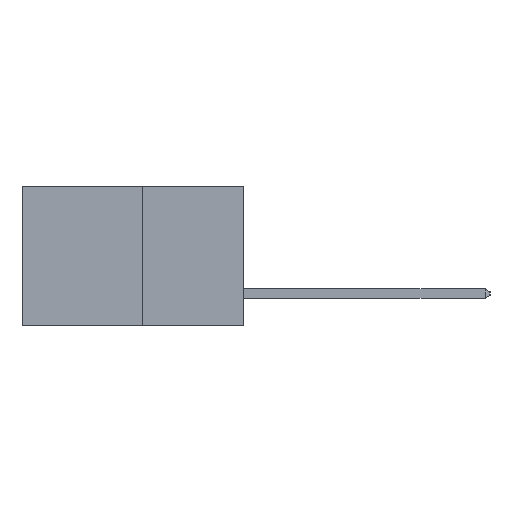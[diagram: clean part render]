
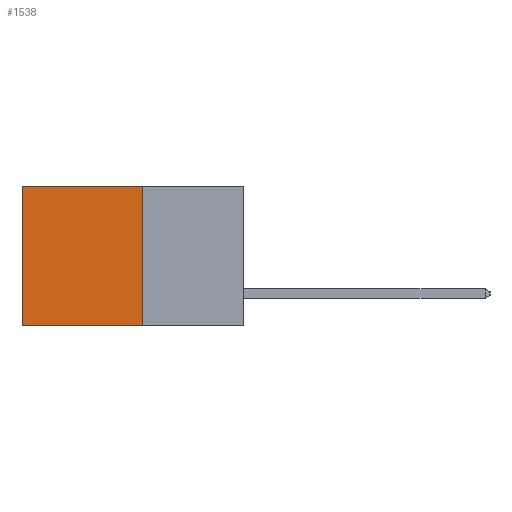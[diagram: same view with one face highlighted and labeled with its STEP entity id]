
A CAD part, left-side view. The second image highlights one B-rep face of the part: STEP entity #1538.
In plain terms, the highlighted planar face has unit normal (-1, 0, 0).
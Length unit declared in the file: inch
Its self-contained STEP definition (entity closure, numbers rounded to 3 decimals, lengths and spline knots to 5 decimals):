
#100 = LINE ( 'NONE', #8875, #11781 ) ;
#270 = CARTESIAN_POINT ( 'NONE',  ( 0.277, 0.27, -0.37 ) ) ;
#289 = CARTESIAN_POINT ( 'NONE',  ( 0.277, 0.59, -0.37 ) ) ;
#321 = DIRECTION ( 'NONE',  ( 0., 1., 0. ) ) ;
#931 = CARTESIAN_POINT ( 'NONE',  ( 0.277, 0.59, 0. ) ) ;
#1231 = CARTESIAN_POINT ( 'NONE',  ( 0.277, 0.27, 0. ) ) ;
#1324 = VERTEX_POINT ( 'NONE', #289 ) ;
#1538 = ADVANCED_FACE ( 'NONE', ( #3487 ), #2249, .F. ) ;
#2160 = CARTESIAN_POINT ( 'NONE',  ( 0.277, 0.27, -0.37 ) ) ;
#2249 = PLANE ( 'NONE',  #11207 ) ;
#3296 = ORIENTED_EDGE ( 'NONE', *, *, #9371, .T. ) ;
#3473 = CARTESIAN_POINT ( 'NONE',  ( 0.277, 0.27, -0.37 ) ) ;
#3487 = FACE_OUTER_BOUND ( 'NONE', #5693, .T. ) ;
#3589 = DIRECTION ( 'NONE',  ( 0., 0., -1. ) ) ;
#3877 = CARTESIAN_POINT ( 'NONE',  ( 0.277, 0.27, 0. ) ) ;
#3900 = DIRECTION ( 'NONE',  ( 0., 0., -1. ) ) ;
#5597 = DIRECTION ( 'NONE',  ( 1., 0., 0. ) ) ;
#5641 = EDGE_CURVE ( 'NONE', #7639, #1324, #5651, .T. ) ;
#5651 = LINE ( 'NONE', #270, #10598 ) ;
#5693 = EDGE_LOOP ( 'NONE', ( #3296, #5935, #12769, #12061 ) ) ;
#5935 = ORIENTED_EDGE ( 'NONE', *, *, #5641, .F. ) ;
#6694 = EDGE_CURVE ( 'NONE', #10848, #10465, #9788, .T. ) ;
#6961 = VECTOR ( 'NONE', #9824, 39.37008 ) ;
#7639 = VERTEX_POINT ( 'NONE', #9329 ) ;
#8875 = CARTESIAN_POINT ( 'NONE',  ( 0.277, 0.59, -0.37 ) ) ;
#9329 = CARTESIAN_POINT ( 'NONE',  ( 0.277, 0.27, -0.37 ) ) ;
#9371 = EDGE_CURVE ( 'NONE', #10465, #1324, #100, .T. ) ;
#9771 = DIRECTION ( 'NONE',  ( 0., 1., 0. ) ) ;
#9788 = LINE ( 'NONE', #1231, #10754 ) ;
#9824 = DIRECTION ( 'NONE',  ( 0., 0., -1. ) ) ;
#10465 = VERTEX_POINT ( 'NONE', #931 ) ;
#10598 = VECTOR ( 'NONE', #321, 39.37008 ) ;
#10754 = VECTOR ( 'NONE', #9771, 39.37008 ) ;
#10848 = VERTEX_POINT ( 'NONE', #3877 ) ;
#11207 = AXIS2_PLACEMENT_3D ( 'NONE', #2160, #5597, #3900 ) ;
#11781 = VECTOR ( 'NONE', #3589, 39.37008 ) ;
#12061 = ORIENTED_EDGE ( 'NONE', *, *, #6694, .T. ) ;
#12494 = LINE ( 'NONE', #3473, #6961 ) ;
#12769 = ORIENTED_EDGE ( 'NONE', *, *, #13177, .F. ) ;
#13177 = EDGE_CURVE ( 'NONE', #10848, #7639, #12494, .T. ) ;
